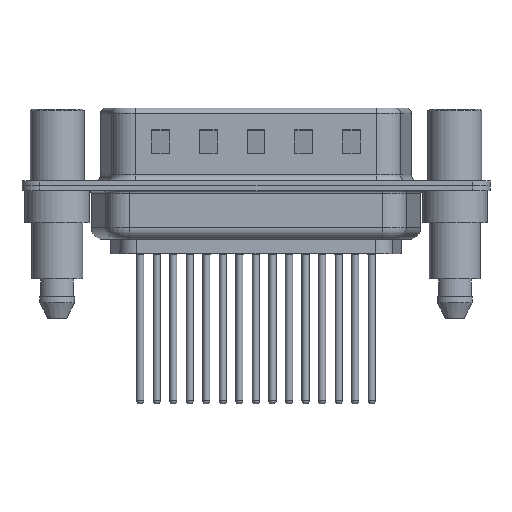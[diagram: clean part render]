
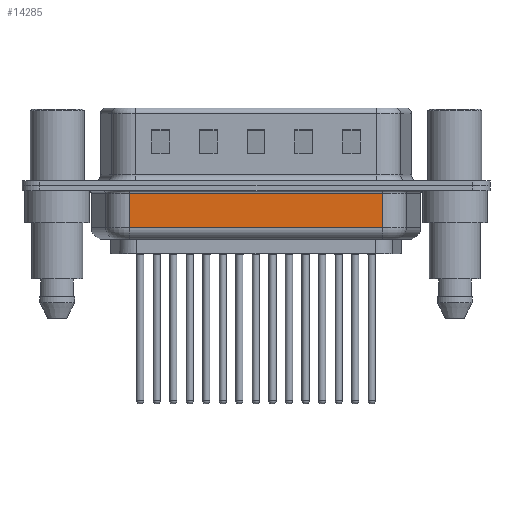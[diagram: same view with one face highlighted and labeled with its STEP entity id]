
A CAD part, front view. The second image highlights one B-rep face of the part: STEP entity #14285.
In plain terms, the highlighted planar face has unit normal (0, -1, 0).
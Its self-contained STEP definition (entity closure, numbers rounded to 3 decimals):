
#698 = ORIENTED_EDGE ( 'NONE', *, *, #17238, .F. ) ;
#872 = EDGE_CURVE ( 'NONE', #3930, #13230, #13602, .T. ) ;
#2292 = VERTEX_POINT ( 'NONE', #9512 ) ;
#2833 = DIRECTION ( 'NONE',  ( 0., 0., 1. ) ) ;
#3091 = CARTESIAN_POINT ( 'NONE',  ( 27.269, -5.35, -4.5 ) ) ;
#3397 = DIRECTION ( 'NONE',  ( -1., 0., 0. ) ) ;
#3578 = CARTESIAN_POINT ( 'NONE',  ( 6.031, -5.35, -3.5 ) ) ;
#3713 = VECTOR ( 'NONE', #16491, 1000. ) ;
#3930 = VERTEX_POINT ( 'NONE', #5016 ) ;
#4686 = CARTESIAN_POINT ( 'NONE',  ( 6.031, -5.35, -3.5 ) ) ;
#4977 = FACE_OUTER_BOUND ( 'NONE', #6657, .T. ) ;
#5016 = CARTESIAN_POINT ( 'NONE',  ( 27.269, -5.35, -3.5 ) ) ;
#5192 = CARTESIAN_POINT ( 'NONE',  ( 27.269, -5.35, -0.65 ) ) ;
#6616 = ORIENTED_EDGE ( 'NONE', *, *, #7625, .T. ) ;
#6657 = EDGE_LOOP ( 'NONE', ( #698, #6616, #10498, #15832 ) ) ;
#6993 = CARTESIAN_POINT ( 'NONE',  ( 6.031, -5.35, -0.65 ) ) ;
#7191 = EDGE_CURVE ( 'NONE', #13230, #2292, #10829, .T. ) ;
#7625 = EDGE_CURVE ( 'NONE', #12722, #3930, #15550, .T. ) ;
#9465 = DIRECTION ( 'NONE',  ( 0., 0., 1. ) ) ;
#9512 = CARTESIAN_POINT ( 'NONE',  ( 6.031, -5.35, -0.65 ) ) ;
#10018 = VECTOR ( 'NONE', #11275, 1000. ) ;
#10138 = CARTESIAN_POINT ( 'NONE',  ( 6.031, -5.35, -4.5 ) ) ;
#10498 = ORIENTED_EDGE ( 'NONE', *, *, #872, .T. ) ;
#10829 = LINE ( 'NONE', #6993, #3713 ) ;
#11275 = DIRECTION ( 'NONE',  ( 1., 0., 0. ) ) ;
#11909 = CARTESIAN_POINT ( 'NONE',  ( 6.031, -5.35, -4.5 ) ) ;
#12269 = LINE ( 'NONE', #11909, #12473 ) ;
#12473 = VECTOR ( 'NONE', #9465, 1000. ) ;
#12722 = VERTEX_POINT ( 'NONE', #4686 ) ;
#12994 = AXIS2_PLACEMENT_3D ( 'NONE', #10138, #14071, #3397 ) ;
#13047 = VECTOR ( 'NONE', #2833, 1000. ) ;
#13230 = VERTEX_POINT ( 'NONE', #5192 ) ;
#13602 = LINE ( 'NONE', #3091, #13047 ) ;
#14071 = DIRECTION ( 'NONE',  ( 0., 1., 0. ) ) ;
#14238 = PLANE ( 'NONE',  #12994 ) ;
#14285 = ADVANCED_FACE ( 'NONE', ( #4977 ), #14238, .F. ) ;
#15550 = LINE ( 'NONE', #3578, #10018 ) ;
#15832 = ORIENTED_EDGE ( 'NONE', *, *, #7191, .T. ) ;
#16491 = DIRECTION ( 'NONE',  ( -1., 0., 0. ) ) ;
#17238 = EDGE_CURVE ( 'NONE', #12722, #2292, #12269, .T. ) ;
